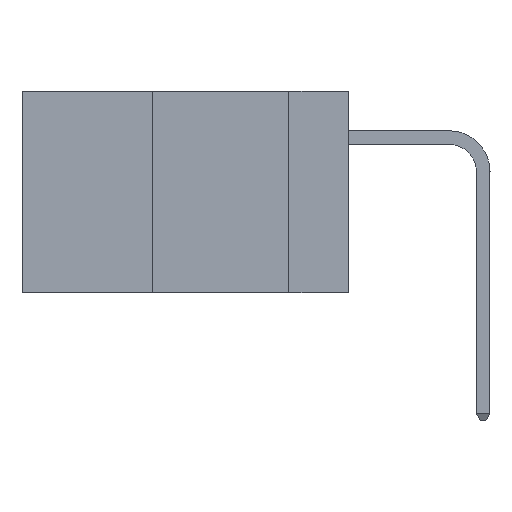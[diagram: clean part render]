
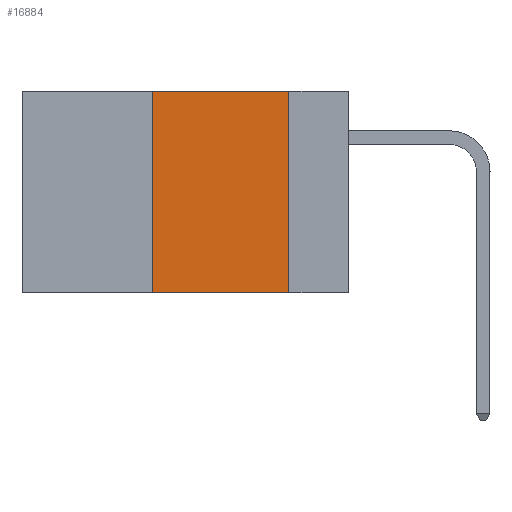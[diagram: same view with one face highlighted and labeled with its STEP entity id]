
A CAD part, left-side view. The second image highlights one B-rep face of the part: STEP entity #16884.
In plain terms, the highlighted planar face has unit normal (-1, 0, 0).
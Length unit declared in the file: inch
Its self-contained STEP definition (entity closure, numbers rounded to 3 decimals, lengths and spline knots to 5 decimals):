
#293 = CARTESIAN_POINT ( 'NONE',  ( 0., 0.11, 0. ) ) ;
#667 = DIRECTION ( 'NONE',  ( 0., -1., 0. ) ) ;
#1366 = LINE ( 'NONE', #13962, #8386 ) ;
#1605 = VERTEX_POINT ( 'NONE', #16255 ) ;
#1628 = ORIENTED_EDGE ( 'NONE', *, *, #17928, .T. ) ;
#2086 = EDGE_LOOP ( 'NONE', ( #4266, #13039, #4052, #1628 ) ) ;
#2115 = LINE ( 'NONE', #17461, #9091 ) ;
#3245 = DIRECTION ( 'NONE',  ( 0., 0., -1. ) ) ;
#4052 = ORIENTED_EDGE ( 'NONE', *, *, #10788, .F. ) ;
#4135 = PLANE ( 'NONE',  #6552 ) ;
#4266 = ORIENTED_EDGE ( 'NONE', *, *, #5718, .F. ) ;
#5523 = CARTESIAN_POINT ( 'NONE',  ( 0., 0.6, 0. ) ) ;
#5718 = EDGE_CURVE ( 'NONE', #14014, #9296, #9144, .T. ) ;
#6401 = CARTESIAN_POINT ( 'NONE',  ( 0., 0.6, 0. ) ) ;
#6552 = AXIS2_PLACEMENT_3D ( 'NONE', #5523, #6922, #16701 ) ;
#6922 = DIRECTION ( 'NONE',  ( 1., 0., 0. ) ) ;
#7811 = DIRECTION ( 'NONE',  ( 0., -1., 0. ) ) ;
#8386 = VECTOR ( 'NONE', #15369, 39.37008 ) ;
#8481 = FACE_OUTER_BOUND ( 'NONE', #2086, .T. ) ;
#9091 = VECTOR ( 'NONE', #667, 39.37008 ) ;
#9144 = LINE ( 'NONE', #17149, #15713 ) ;
#9296 = VERTEX_POINT ( 'NONE', #13677 ) ;
#10240 = CARTESIAN_POINT ( 'NONE',  ( 0., 0.36, -0.37 ) ) ;
#10788 = EDGE_CURVE ( 'NONE', #14634, #1605, #1366, .T. ) ;
#13039 = ORIENTED_EDGE ( 'NONE', *, *, #16023, .F. ) ;
#13677 = CARTESIAN_POINT ( 'NONE',  ( 0., 0.11, -0.37 ) ) ;
#13962 = CARTESIAN_POINT ( 'NONE',  ( 0., 0.36, 0. ) ) ;
#14014 = VERTEX_POINT ( 'NONE', #293 ) ;
#14634 = VERTEX_POINT ( 'NONE', #10240 ) ;
#15369 = DIRECTION ( 'NONE',  ( 0., 0., 1. ) ) ;
#15713 = VECTOR ( 'NONE', #3245, 39.37008 ) ;
#16023 = EDGE_CURVE ( 'NONE', #1605, #14014, #17268, .T. ) ;
#16255 = CARTESIAN_POINT ( 'NONE',  ( 0., 0.36, 0. ) ) ;
#16701 = DIRECTION ( 'NONE',  ( 0., 0., -1. ) ) ;
#16814 = VECTOR ( 'NONE', #7811, 39.37008 ) ;
#16884 = ADVANCED_FACE ( 'NONE', ( #8481 ), #4135, .F. ) ;
#17149 = CARTESIAN_POINT ( 'NONE',  ( 0., 0.11, 0. ) ) ;
#17268 = LINE ( 'NONE', #6401, #16814 ) ;
#17461 = CARTESIAN_POINT ( 'NONE',  ( 0., 0.6, -0.37 ) ) ;
#17928 = EDGE_CURVE ( 'NONE', #14634, #9296, #2115, .T. ) ;
